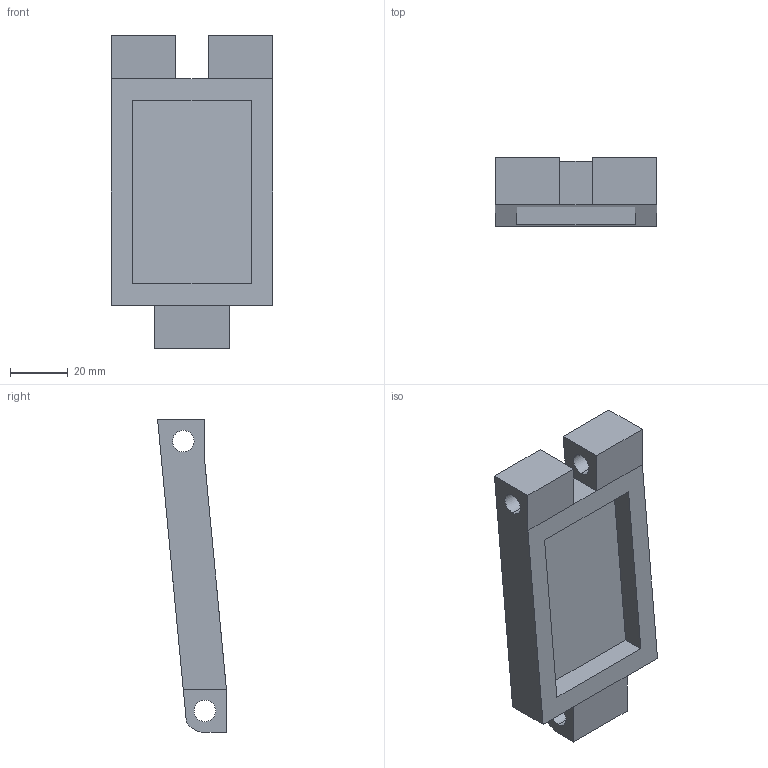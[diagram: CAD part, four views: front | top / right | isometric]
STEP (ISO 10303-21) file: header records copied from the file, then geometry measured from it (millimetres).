
FILE_DESCRIPTION (( 'STEP AP203' ), '1' );
FILE_NAME ('Top.STEP', '2013-09-22T12:18:46', ( '' ), ( '' ), 'SwSTEP 2.0', 'SolidWorks 2013', '' );
FILE_SCHEMA (( 'CONFIG_CONTROL_DESIGN' ));
Length unit declared in the file: millimetre
Products named in the file (1): Top
Bounding box: 56.25 x 23.93 x 108.75 mm (x, y, z)
Volume: 59624.3 mm3; surface area: 19414.8 mm2
Topology: 1 solids, 1 shells, 29 faces, 74 edges, 48 vertices
Faces by surface type: plane 22, cylinder 7
Entity records: 959 total; most frequent: CARTESIAN_POINT 152, DIRECTION 148, ORIENTED_EDGE 148, EDGE_CURVE 74, VECTOR 60, LINE 60, VERTEX_POINT 48, AXIS2_PLACEMENT_3D 44
